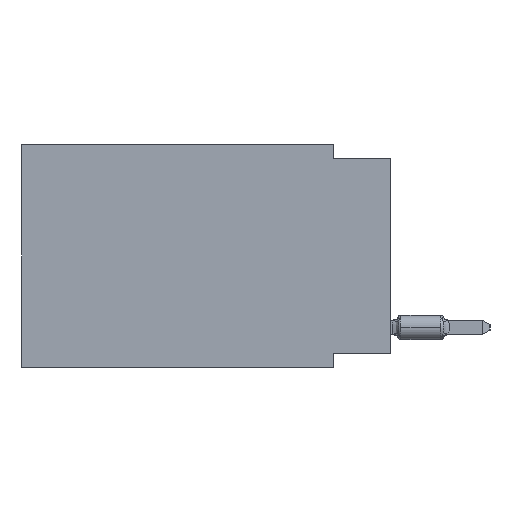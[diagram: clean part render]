
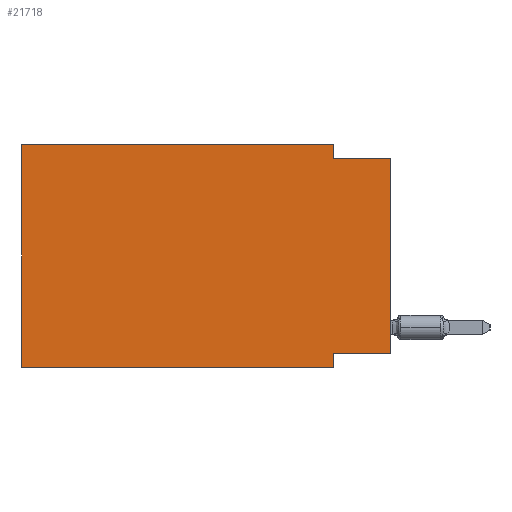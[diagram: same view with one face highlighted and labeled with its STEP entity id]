
A CAD part, left-side view. The second image highlights one B-rep face of the part: STEP entity #21718.
In plain terms, the highlighted planar face has unit normal (-1, 0, 0).
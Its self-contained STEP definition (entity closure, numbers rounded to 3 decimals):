
#414 = FACE_OUTER_BOUND ( 'NONE', #20304, .T. ) ;
#1202 = DIRECTION ( 'NONE',  ( 0., -1., 0. ) ) ;
#1740 = EDGE_CURVE ( 'NONE', #25758, #8904, #12492, .T. ) ;
#2526 = VECTOR ( 'NONE', #12734, 1000. ) ;
#2967 = ORIENTED_EDGE ( 'NONE', *, *, #7907, .F. ) ;
#3007 = ORIENTED_EDGE ( 'NONE', *, *, #1740, .F. ) ;
#3231 = VERTEX_POINT ( 'NONE', #21408 ) ;
#3759 = EDGE_CURVE ( 'NONE', #8001, #3231, #16112, .T. ) ;
#5129 = VERTEX_POINT ( 'NONE', #15041 ) ;
#5498 = ORIENTED_EDGE ( 'NONE', *, *, #3759, .F. ) ;
#6151 = VERTEX_POINT ( 'NONE', #12662 ) ;
#6367 = CARTESIAN_POINT ( 'NONE',  ( 0., 0., -0.635 ) ) ;
#6636 = ORIENTED_EDGE ( 'NONE', *, *, #17500, .T. ) ;
#7085 = EDGE_CURVE ( 'NONE', #8904, #25405, #20690, .T. ) ;
#7166 = CARTESIAN_POINT ( 'NONE',  ( 0., 16.383, 0. ) ) ;
#7292 = VECTOR ( 'NONE', #1202, 1000. ) ;
#7907 = EDGE_CURVE ( 'NONE', #15929, #25758, #10084, .T. ) ;
#8001 = VERTEX_POINT ( 'NONE', #27257 ) ;
#8757 = ORIENTED_EDGE ( 'NONE', *, *, #16831, .F. ) ;
#8904 = VERTEX_POINT ( 'NONE', #14779 ) ;
#9505 = EDGE_CURVE ( 'NONE', #6151, #25405, #15874, .T. ) ;
#9544 = CARTESIAN_POINT ( 'NONE',  ( 0., 0., 0. ) ) ;
#10084 = LINE ( 'NONE', #11915, #7292 ) ;
#10944 = VECTOR ( 'NONE', #14728, 1000. ) ;
#11299 = AXIS2_PLACEMENT_3D ( 'NONE', #7166, #23957, #24371 ) ;
#11385 = DIRECTION ( 'NONE',  ( 0., 0., 1. ) ) ;
#11915 = CARTESIAN_POINT ( 'NONE',  ( 0., 16.383, 0. ) ) ;
#12144 = CARTESIAN_POINT ( 'NONE',  ( 0., 2.54, 0. ) ) ;
#12492 = LINE ( 'NONE', #25989, #21420 ) ;
#12662 = CARTESIAN_POINT ( 'NONE',  ( 0., 0., -9.271 ) ) ;
#12734 = DIRECTION ( 'NONE',  ( 0., -1., 0. ) ) ;
#13103 = PLANE ( 'NONE',  #11299 ) ;
#13830 = ORIENTED_EDGE ( 'NONE', *, *, #9505, .T. ) ;
#13987 = CARTESIAN_POINT ( 'NONE',  ( 0., 16.383, 0. ) ) ;
#14346 = CARTESIAN_POINT ( 'NONE',  ( 0., 0., -0.635 ) ) ;
#14580 = LINE ( 'NONE', #14708, #16968 ) ;
#14708 = CARTESIAN_POINT ( 'NONE',  ( 0., 0., -9.271 ) ) ;
#14728 = DIRECTION ( 'NONE',  ( 0., 0., 1. ) ) ;
#14779 = CARTESIAN_POINT ( 'NONE',  ( 0., 2.54, -0.635 ) ) ;
#14834 = LINE ( 'NONE', #18947, #2526 ) ;
#14839 = DIRECTION ( 'NONE',  ( 0., 1., 0. ) ) ;
#15041 = CARTESIAN_POINT ( 'NONE',  ( 0., 16.383, -9.906 ) ) ;
#15874 = LINE ( 'NONE', #9544, #25781 ) ;
#15929 = VERTEX_POINT ( 'NONE', #13987 ) ;
#16112 = LINE ( 'NONE', #18246, #20140 ) ;
#16249 = VECTOR ( 'NONE', #23347, 1000. ) ;
#16831 = EDGE_CURVE ( 'NONE', #6151, #8001, #14580, .T. ) ;
#16863 = CARTESIAN_POINT ( 'NONE',  ( 0., 16.383, 0. ) ) ;
#16968 = VECTOR ( 'NONE', #14839, 1000. ) ;
#17500 = EDGE_CURVE ( 'NONE', #5129, #3231, #14834, .T. ) ;
#18079 = ORIENTED_EDGE ( 'NONE', *, *, #23628, .F. ) ;
#18246 = CARTESIAN_POINT ( 'NONE',  ( 0., 2.54, -9.906 ) ) ;
#18947 = CARTESIAN_POINT ( 'NONE',  ( 0., 16.383, -9.906 ) ) ;
#19282 = ORIENTED_EDGE ( 'NONE', *, *, #7085, .F. ) ;
#20140 = VECTOR ( 'NONE', #26825, 1000. ) ;
#20304 = EDGE_LOOP ( 'NONE', ( #13830, #19282, #3007, #2967, #18079, #6636, #5498, #8757 ) ) ;
#20690 = LINE ( 'NONE', #14346, #16249 ) ;
#21408 = CARTESIAN_POINT ( 'NONE',  ( 0., 2.54, -9.906 ) ) ;
#21420 = VECTOR ( 'NONE', #26655, 1000. ) ;
#21718 = ADVANCED_FACE ( 'NONE', ( #414 ), #13103, .F. ) ;
#23347 = DIRECTION ( 'NONE',  ( 0., -1., 0. ) ) ;
#23628 = EDGE_CURVE ( 'NONE', #5129, #15929, #27570, .T. ) ;
#23957 = DIRECTION ( 'NONE',  ( 1., 0., 0. ) ) ;
#24371 = DIRECTION ( 'NONE',  ( 0., 0., -1. ) ) ;
#25405 = VERTEX_POINT ( 'NONE', #6367 ) ;
#25758 = VERTEX_POINT ( 'NONE', #12144 ) ;
#25781 = VECTOR ( 'NONE', #11385, 1000. ) ;
#25989 = CARTESIAN_POINT ( 'NONE',  ( 0., 2.54, 0. ) ) ;
#26655 = DIRECTION ( 'NONE',  ( 0., 0., -1. ) ) ;
#26825 = DIRECTION ( 'NONE',  ( 0., 0., -1. ) ) ;
#27257 = CARTESIAN_POINT ( 'NONE',  ( 0., 2.54, -9.271 ) ) ;
#27570 = LINE ( 'NONE', #16863, #10944 ) ;
